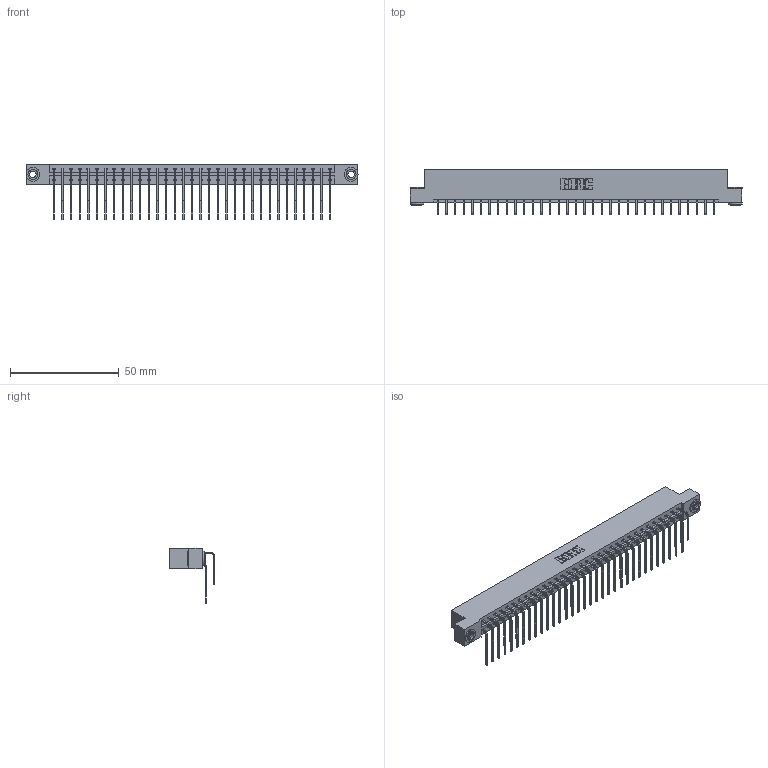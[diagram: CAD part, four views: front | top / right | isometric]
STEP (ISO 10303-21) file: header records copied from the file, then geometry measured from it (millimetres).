
FILE_DESCRIPTION (( 'STEP AP203' ), '1' );
FILE_NAME ('833-066-559-203.STEP', '2020-06-05T09:41:36', ( '' ), ( '' ), 'SwSTEP 2.0', 'SolidWorks 2020', '' );
FILE_SCHEMA (( 'CONFIG_CONTROL_DESIGN' ));
Length unit declared in the file: inch
Products named in the file (5): 345-250-002_345-250-002-102; 833-066-559-203; 833 Part_Flush - .156 Dia - TH; 345-292-001_559 Tail - 2; 345-292-001_558 559 Tail - 1
Assembly tree (69 placements, depth 2):
  833-066-559-203
    833 Part_Flush - .156 Dia - TH
    345-292-001_558 559 Tail - 1  x33
    345-292-001_559 Tail - 2  x33
    345-250-002_345-250-002-102  x2
Bounding box: 152.3 x 20.9 x 25.53 mm (x, y, z)
Volume: 15864.8 mm3; surface area: 20776.7 mm2
Topology: 69 solids, 69 shells, 3716 faces, 11013 edges, 7250 vertices
Faces by surface type: plane 2588, cylinder 1120, cone 8
Entity records: 24828 total; most frequent: CARTESIAN_POINT 4152, ORIENTED_EDGE 4030, DIRECTION 3577, EDGE_CURVE 2015, LINE 1823, VECTOR 1823, VERTEX_POINT 1338, AXIS2_PLACEMENT_3D 877
